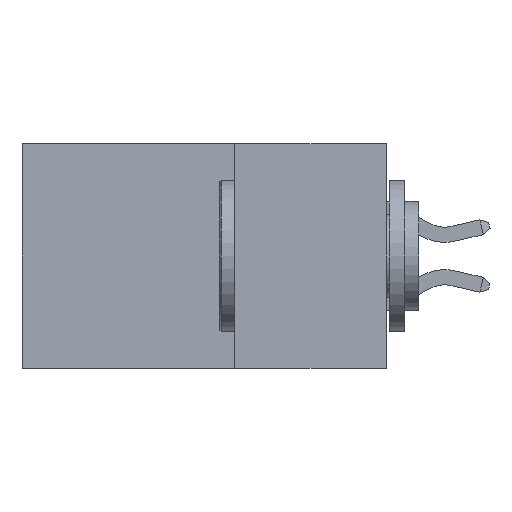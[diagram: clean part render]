
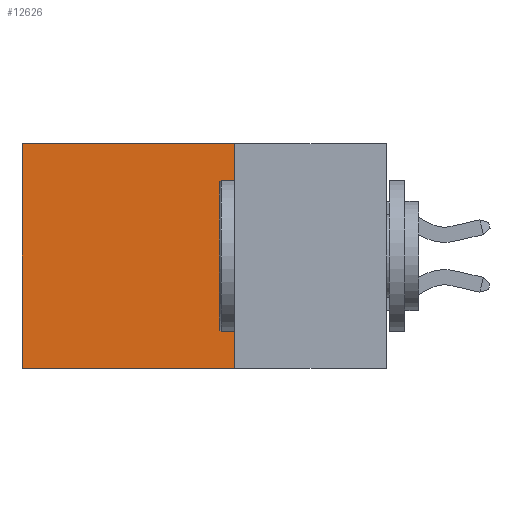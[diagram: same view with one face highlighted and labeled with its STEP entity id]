
A CAD part, left-side view. The second image highlights one B-rep face of the part: STEP entity #12626.
In plain terms, the highlighted planar face has unit normal (-1, 0, 0).
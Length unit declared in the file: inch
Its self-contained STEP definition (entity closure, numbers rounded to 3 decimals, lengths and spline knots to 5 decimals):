
#590 = LINE ( 'NONE', #4641, #4221 ) ;
#655 = EDGE_CURVE ( 'NONE', #19274, #14451, #4745, .T. ) ;
#715 = EDGE_CURVE ( 'NONE', #14493, #7611, #19107, .T. ) ;
#999 = DIRECTION ( 'NONE',  ( 0., 0., -1. ) ) ;
#1906 = ORIENTED_EDGE ( 'NONE', *, *, #655, .F. ) ;
#2179 = DIRECTION ( 'NONE',  ( 0., 0., -1. ) ) ;
#3680 = CARTESIAN_POINT ( 'NONE',  ( 0.298, 0.25, 0. ) ) ;
#4128 = CARTESIAN_POINT ( 'NONE',  ( 0.298, 0.6, 0. ) ) ;
#4221 = VECTOR ( 'NONE', #6211, 39.37008 ) ;
#4641 = CARTESIAN_POINT ( 'NONE',  ( 0.298, 0.25, -0.37 ) ) ;
#4745 = LINE ( 'NONE', #18709, #8371 ) ;
#4747 = LINE ( 'NONE', #15370, #8861 ) ;
#6171 = DIRECTION ( 'NONE',  ( 0., 1., 0. ) ) ;
#6211 = DIRECTION ( 'NONE',  ( 0., 1., 0. ) ) ;
#7084 = CARTESIAN_POINT ( 'NONE',  ( 0.298, 0.6, -0.37 ) ) ;
#7243 = CARTESIAN_POINT ( 'NONE',  ( 0.298, 0.25, 0. ) ) ;
#7611 = VERTEX_POINT ( 'NONE', #7084 ) ;
#8206 = FACE_OUTER_BOUND ( 'NONE', #18824, .T. ) ;
#8371 = VECTOR ( 'NONE', #10463, 39.37008 ) ;
#8384 = PLANE ( 'NONE',  #9826 ) ;
#8861 = VECTOR ( 'NONE', #6171, 39.37008 ) ;
#9826 = AXIS2_PLACEMENT_3D ( 'NONE', #3680, #11491, #2179 ) ;
#10463 = DIRECTION ( 'NONE',  ( 0., 0., -1. ) ) ;
#11491 = DIRECTION ( 'NONE',  ( 1., 0., 0. ) ) ;
#12626 = ADVANCED_FACE ( 'NONE', ( #8206 ), #8384, .F. ) ;
#13402 = CARTESIAN_POINT ( 'NONE',  ( 0.298, 0.25, -0.37 ) ) ;
#14271 = EDGE_CURVE ( 'NONE', #19274, #14493, #4747, .T. ) ;
#14451 = VERTEX_POINT ( 'NONE', #13402 ) ;
#14493 = VERTEX_POINT ( 'NONE', #16613 ) ;
#14620 = EDGE_CURVE ( 'NONE', #14451, #7611, #590, .T. ) ;
#15097 = VECTOR ( 'NONE', #999, 39.37008 ) ;
#15370 = CARTESIAN_POINT ( 'NONE',  ( 0.298, 0.25, 0. ) ) ;
#16613 = CARTESIAN_POINT ( 'NONE',  ( 0.298, 0.6, 0. ) ) ;
#16847 = ORIENTED_EDGE ( 'NONE', *, *, #715, .T. ) ;
#17596 = ORIENTED_EDGE ( 'NONE', *, *, #14271, .T. ) ;
#18709 = CARTESIAN_POINT ( 'NONE',  ( 0.298, 0.25, 0. ) ) ;
#18824 = EDGE_LOOP ( 'NONE', ( #16847, #19830, #1906, #17596 ) ) ;
#19107 = LINE ( 'NONE', #4128, #15097 ) ;
#19274 = VERTEX_POINT ( 'NONE', #7243 ) ;
#19830 = ORIENTED_EDGE ( 'NONE', *, *, #14620, .F. ) ;
